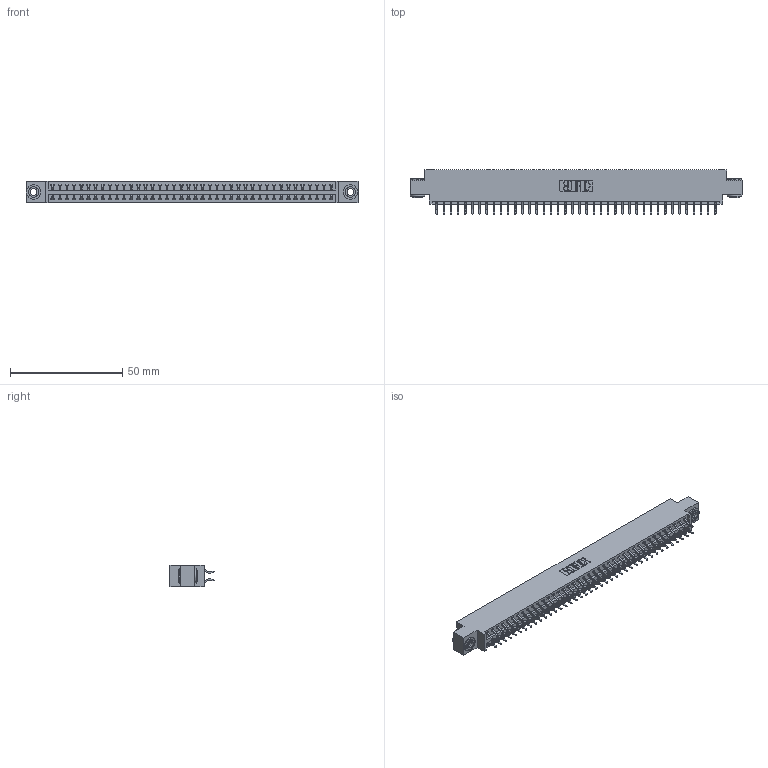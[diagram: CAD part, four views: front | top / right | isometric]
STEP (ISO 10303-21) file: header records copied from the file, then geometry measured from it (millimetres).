
FILE_DESCRIPTION (( 'STEP AP203' ), '1' );
FILE_NAME ('346-080-556-803.STEP', '2022-05-25T16:23:18', ( '' ), ( '' ), 'SwSTEP 2.0', 'SolidWorks 2020', '' );
FILE_SCHEMA (( 'CONFIG_CONTROL_DESIGN' ));
Length unit declared in the file: inch
Products named in the file (4): 345-250-002_345-250-002-102; 346 Part_0.170 Offset - 0.156 Dia-TH; 345-292-001_556 Tail; 346-080-556-803
Assembly tree (83 placements, depth 2):
  346-080-556-803
    346 Part_0.170 Offset - 0.156 Dia-TH
    345-292-001_556 Tail  x80
    345-250-002_345-250-002-102  x2
Bounding box: 147.57 x 19.57 x 9.4 mm (x, y, z)
Volume: 14218.3 mm3; surface area: 19866.6 mm2
Topology: 83 solids, 83 shells, 4818 faces, 14293 edges, 9418 vertices
Faces by surface type: plane 3224, cylinder 1586, cone 8
Entity records: 27792 total; most frequent: CARTESIAN_POINT 4581, ORIENTED_EDGE 4494, DIRECTION 4105, EDGE_CURVE 2247, VECTOR 1923, LINE 1923, VERTEX_POINT 1494, AXIS2_PLACEMENT_3D 1091
